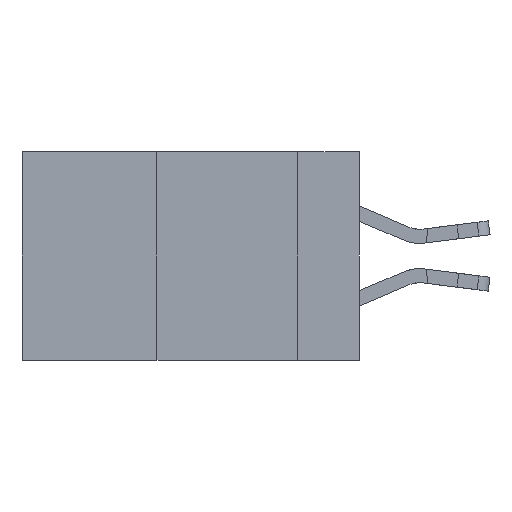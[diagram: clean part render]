
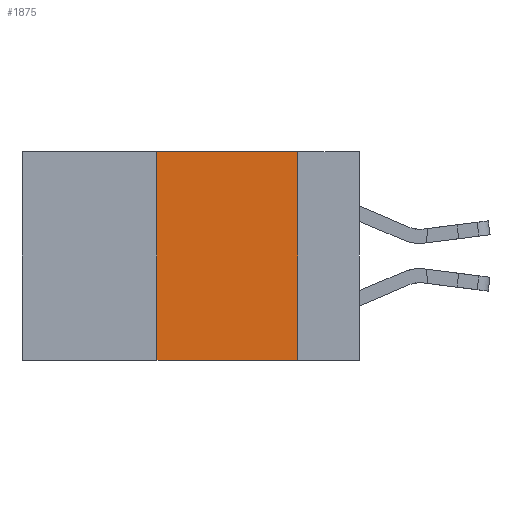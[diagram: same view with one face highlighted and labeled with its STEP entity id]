
A CAD part, left-side view. The second image highlights one B-rep face of the part: STEP entity #1875.
In plain terms, the highlighted planar face has unit normal (-1, 0, 0).
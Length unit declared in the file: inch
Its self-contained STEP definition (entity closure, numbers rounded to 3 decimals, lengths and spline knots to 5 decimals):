
#670 = EDGE_LOOP ( 'NONE', ( #2866, #2748, #13445, #8103 ) ) ;
#1353 = EDGE_CURVE ( 'NONE', #2448, #4308, #7693, .T. ) ;
#1684 = CARTESIAN_POINT ( 'NONE',  ( 0., 0.11, -0.37 ) ) ;
#1875 = ADVANCED_FACE ( 'NONE', ( #6347 ), #12970, .F. ) ;
#2109 = CARTESIAN_POINT ( 'NONE',  ( 0., 0.11, 0. ) ) ;
#2417 = VECTOR ( 'NONE', #9222, 39.37008 ) ;
#2448 = VERTEX_POINT ( 'NONE', #5112 ) ;
#2730 = CARTESIAN_POINT ( 'NONE',  ( 0., 0.36, 0. ) ) ;
#2748 = ORIENTED_EDGE ( 'NONE', *, *, #10478, .F. ) ;
#2866 = ORIENTED_EDGE ( 'NONE', *, *, #3453, .F. ) ;
#3453 = EDGE_CURVE ( 'NONE', #11291, #11515, #8745, .T. ) ;
#3458 = DIRECTION ( 'NONE',  ( 0., -1., 0. ) ) ;
#4308 = VERTEX_POINT ( 'NONE', #2730 ) ;
#4716 = DIRECTION ( 'NONE',  ( 1., 0., 0. ) ) ;
#5112 = CARTESIAN_POINT ( 'NONE',  ( 0., 0.36, -0.37 ) ) ;
#5717 = LINE ( 'NONE', #12547, #20571 ) ;
#6347 = FACE_OUTER_BOUND ( 'NONE', #670, .T. ) ;
#7693 = LINE ( 'NONE', #20983, #2417 ) ;
#8027 = VECTOR ( 'NONE', #3458, 39.37008 ) ;
#8103 = ORIENTED_EDGE ( 'NONE', *, *, #9685, .T. ) ;
#8244 = CARTESIAN_POINT ( 'NONE',  ( 0., 0.6, -0.37 ) ) ;
#8458 = LINE ( 'NONE', #8244, #8027 ) ;
#8745 = LINE ( 'NONE', #2109, #18864 ) ;
#9222 = DIRECTION ( 'NONE',  ( 0., 0., 1. ) ) ;
#9685 = EDGE_CURVE ( 'NONE', #2448, #11515, #8458, .T. ) ;
#10478 = EDGE_CURVE ( 'NONE', #4308, #11291, #5717, .T. ) ;
#11123 = AXIS2_PLACEMENT_3D ( 'NONE', #19615, #4716, #16350 ) ;
#11291 = VERTEX_POINT ( 'NONE', #15749 ) ;
#11515 = VERTEX_POINT ( 'NONE', #1684 ) ;
#12547 = CARTESIAN_POINT ( 'NONE',  ( 0., 0.6, 0. ) ) ;
#12970 = PLANE ( 'NONE',  #11123 ) ;
#13445 = ORIENTED_EDGE ( 'NONE', *, *, #1353, .F. ) ;
#15749 = CARTESIAN_POINT ( 'NONE',  ( 0., 0.11, 0. ) ) ;
#16350 = DIRECTION ( 'NONE',  ( 0., 0., -1. ) ) ;
#17147 = DIRECTION ( 'NONE',  ( 0., 0., -1. ) ) ;
#18864 = VECTOR ( 'NONE', #17147, 39.37008 ) ;
#19194 = DIRECTION ( 'NONE',  ( 0., -1., 0. ) ) ;
#19615 = CARTESIAN_POINT ( 'NONE',  ( 0., 0.6, 0. ) ) ;
#20571 = VECTOR ( 'NONE', #19194, 39.37008 ) ;
#20983 = CARTESIAN_POINT ( 'NONE',  ( 0., 0.36, 0. ) ) ;
